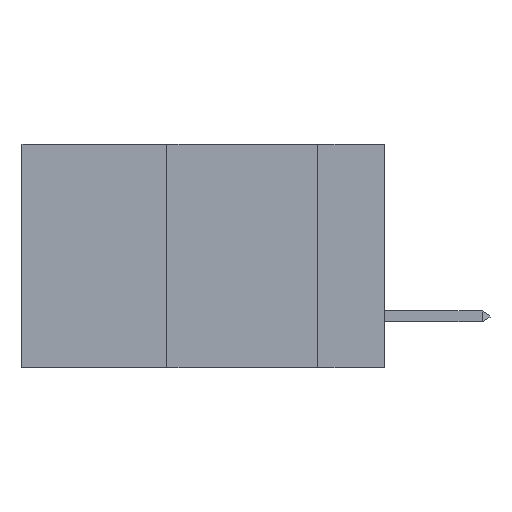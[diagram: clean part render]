
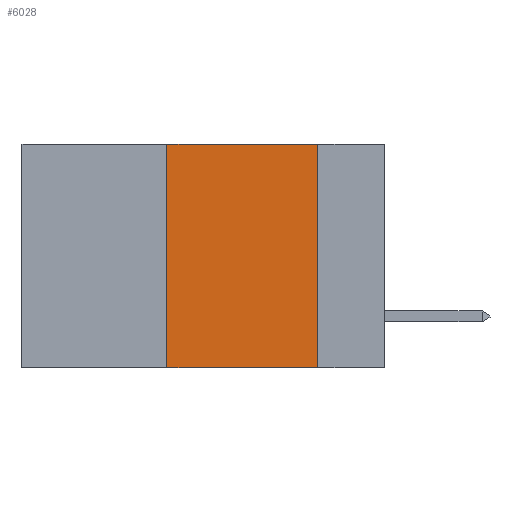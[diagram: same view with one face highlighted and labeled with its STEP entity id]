
A CAD part, left-side view. The second image highlights one B-rep face of the part: STEP entity #6028.
In plain terms, the highlighted planar face has unit normal (-1, 0, 0).
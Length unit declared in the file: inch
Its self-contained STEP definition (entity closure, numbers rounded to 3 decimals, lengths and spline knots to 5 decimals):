
#44 = LINE ( 'NONE', #8967, #6793 ) ;
#155 = CARTESIAN_POINT ( 'NONE',  ( 0., 0.36, -0.37 ) ) ;
#902 = ORIENTED_EDGE ( 'NONE', *, *, #28102, .F. ) ;
#1716 = DIRECTION ( 'NONE',  ( 0., 0., -1. ) ) ;
#2374 = VECTOR ( 'NONE', #3280, 39.37008 ) ;
#3280 = DIRECTION ( 'NONE',  ( 0., 0., 1. ) ) ;
#4805 = DIRECTION ( 'NONE',  ( 0., -1., 0. ) ) ;
#5161 = CARTESIAN_POINT ( 'NONE',  ( 0., 0.11, 0. ) ) ;
#5275 = ORIENTED_EDGE ( 'NONE', *, *, #8838, .F. ) ;
#6028 = ADVANCED_FACE ( 'NONE', ( #30046 ), #28708, .F. ) ;
#6793 = VECTOR ( 'NONE', #13958, 39.37008 ) ;
#8817 = DIRECTION ( 'NONE',  ( 0., 0., -1. ) ) ;
#8838 = EDGE_CURVE ( 'NONE', #20544, #15377, #11066, .T. ) ;
#8967 = CARTESIAN_POINT ( 'NONE',  ( 0., 0.6, -0.37 ) ) ;
#11066 = LINE ( 'NONE', #12321, #16911 ) ;
#11154 = AXIS2_PLACEMENT_3D ( 'NONE', #14159, #16676, #1716 ) ;
#11404 = ORIENTED_EDGE ( 'NONE', *, *, #28904, .F. ) ;
#12321 = CARTESIAN_POINT ( 'NONE',  ( 0., 0.6, 0. ) ) ;
#13325 = ORIENTED_EDGE ( 'NONE', *, *, #21103, .T. ) ;
#13958 = DIRECTION ( 'NONE',  ( 0., -1., 0. ) ) ;
#14159 = CARTESIAN_POINT ( 'NONE',  ( 0., 0.6, 0. ) ) ;
#15377 = VERTEX_POINT ( 'NONE', #5161 ) ;
#15708 = CARTESIAN_POINT ( 'NONE',  ( 0., 0.36, 0. ) ) ;
#16442 = LINE ( 'NONE', #15708, #2374 ) ;
#16676 = DIRECTION ( 'NONE',  ( 1., 0., 0. ) ) ;
#16911 = VECTOR ( 'NONE', #4805, 39.37008 ) ;
#17133 = LINE ( 'NONE', #18770, #31498 ) ;
#18770 = CARTESIAN_POINT ( 'NONE',  ( 0., 0.11, 0. ) ) ;
#19178 = CARTESIAN_POINT ( 'NONE',  ( 0., 0.36, 0. ) ) ;
#19433 = VERTEX_POINT ( 'NONE', #155 ) ;
#20544 = VERTEX_POINT ( 'NONE', #19178 ) ;
#21103 = EDGE_CURVE ( 'NONE', #19433, #22023, #44, .T. ) ;
#22023 = VERTEX_POINT ( 'NONE', #27791 ) ;
#27791 = CARTESIAN_POINT ( 'NONE',  ( 0., 0.11, -0.37 ) ) ;
#28102 = EDGE_CURVE ( 'NONE', #19433, #20544, #16442, .T. ) ;
#28708 = PLANE ( 'NONE',  #11154 ) ;
#28888 = EDGE_LOOP ( 'NONE', ( #11404, #5275, #902, #13325 ) ) ;
#28904 = EDGE_CURVE ( 'NONE', #15377, #22023, #17133, .T. ) ;
#30046 = FACE_OUTER_BOUND ( 'NONE', #28888, .T. ) ;
#31498 = VECTOR ( 'NONE', #8817, 39.37008 ) ;
